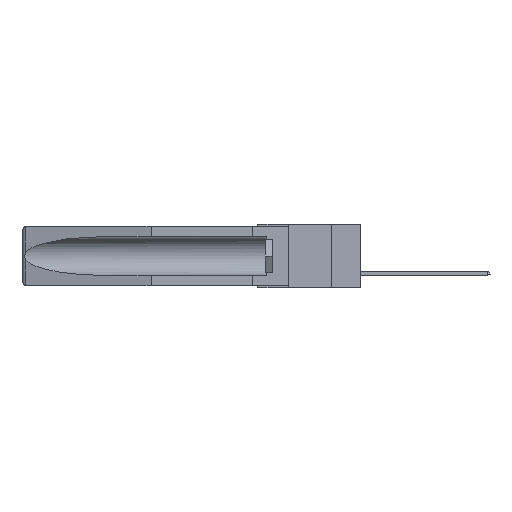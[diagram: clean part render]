
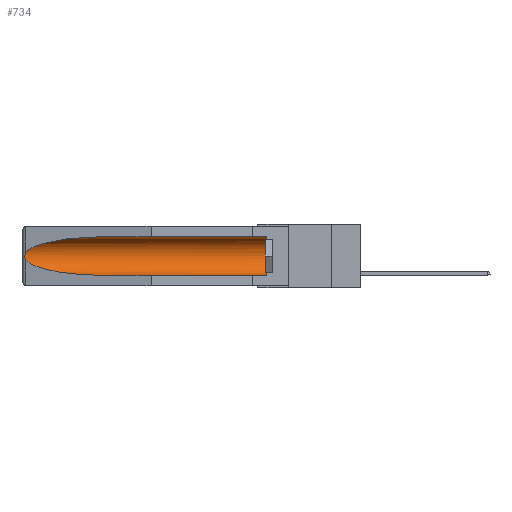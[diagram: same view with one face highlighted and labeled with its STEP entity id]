
A CAD part, left-side view. The second image highlights one B-rep face of the part: STEP entity #734.
In plain terms, the highlighted cylindrical face has radius 2.857 mm (diameter 5.715 mm), a partial arc.
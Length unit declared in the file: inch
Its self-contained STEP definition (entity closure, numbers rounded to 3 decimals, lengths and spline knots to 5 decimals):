
#671 = EDGE_CURVE ( 'NONE', #20543, #9128, #11308, .T. ) ;
#721 = CARTESIAN_POINT ( 'NONE',  ( 0.26537, 1.52718, -0.19328 ) ) ;
#734 = ADVANCED_FACE ( 'NONE', ( #20294 ), #13253, .F. ) ;
#938 = CARTESIAN_POINT ( 'NONE',  ( 0.21114, 1.30732, -0.059 ) ) ;
#1010 =( BOUNDED_CURVE ( )  B_SPLINE_CURVE ( 3, ( #13938, #18757, #17232, #10865 ),
 .UNSPECIFIED., .F., .T. ) 
 B_SPLINE_CURVE_WITH_KNOTS ( ( 4, 4 ),
 ( 0.1948, 1.5708 ),
 .UNSPECIFIED. ) 
 CURVE ( )  GEOMETRIC_REPRESENTATION_ITEM ( )  RATIONAL_B_SPLINE_CURVE ( ( 1., 0.848, 0.848, 1. ) ) 
 REPRESENTATION_ITEM ( '' )  );
#1657 = EDGE_CURVE ( 'NONE', #9608, #5144, #15393, .T. ) ;
#1687 = CARTESIAN_POINT ( 'NONE',  ( 0.26597, 1.52961, -0.15275 ) ) ;
#2240 = CARTESIAN_POINT ( 'NONE',  ( 0.155, -0.30754, -0.1715 ) ) ;
#2378 = VERTEX_POINT ( 'NONE', #11869 ) ;
#2983 = AXIS2_PLACEMENT_3D ( 'NONE', #6679, #3590, #8170 ) ;
#3305 = CARTESIAN_POINT ( 'NONE',  ( 0.26654, 1.53092, -0.15636 ) ) ;
#3590 = DIRECTION ( 'NONE',  ( 0., -1., 0. ) ) ;
#3650 = DIRECTION ( 'NONE',  ( 0., 0., 1. ) ) ;
#3993 = ORIENTED_EDGE ( 'NONE', *, *, #13412, .T. ) ;
#4136 = ORIENTED_EDGE ( 'NONE', *, *, #8612, .F. ) ;
#4415 = CARTESIAN_POINT ( 'NONE',  ( 0.155, -0.30754, -0.284 ) ) ;
#5022 = CIRCLE ( 'NONE', #2983, 0.1125 ) ;
#5144 = VERTEX_POINT ( 'NONE', #10564 ) ;
#6501 = VECTOR ( 'NONE', #14808, 39.37008 ) ;
#6592 = VECTOR ( 'NONE', #14310, 39.37008 ) ;
#6679 = CARTESIAN_POINT ( 'NONE',  ( 0.155, 0.126, -0.1715 ) ) ;
#7323 = ORIENTED_EDGE ( 'NONE', *, *, #671, .T. ) ;
#8170 = DIRECTION ( 'NONE',  ( 0., 0., 1. ) ) ;
#8325 = VERTEX_POINT ( 'NONE', #18918 ) ;
#8612 = EDGE_CURVE ( 'NONE', #8325, #2378, #20167, .T. ) ;
#8706 = CARTESIAN_POINT ( 'NONE',  ( 0.2673, 1.53269, -0.17917 ) ) ;
#9128 = VERTEX_POINT ( 'NONE', #16976 ) ;
#9608 = VERTEX_POINT ( 'NONE', #13157 ) ;
#10125 = CARTESIAN_POINT ( 'NONE',  ( 0.26597, 1.5296, -0.19026 ) ) ;
#10564 = CARTESIAN_POINT ( 'NONE',  ( 0.26537, 1.52718, -0.19328 ) ) ;
#10618 = ORIENTED_EDGE ( 'NONE', *, *, #1657, .T. ) ;
#10779 = EDGE_LOOP ( 'NONE', ( #13760, #10618, #15828, #4136, #3993, #7323 ) ) ;
#10865 = CARTESIAN_POINT ( 'NONE',  ( 0.155, 1.07973, -0.284 ) ) ;
#11308 = LINE ( 'NONE', #11812, #6501 ) ;
#11812 = CARTESIAN_POINT ( 'NONE',  ( 0.155, -0.30754, -0.059 ) ) ;
#11869 = CARTESIAN_POINT ( 'NONE',  ( 0.155, 1.07973, -0.284 ) ) ;
#12294 = CARTESIAN_POINT ( 'NONE',  ( 0.26537, 1.52718, -0.14972 ) ) ;
#13157 = CARTESIAN_POINT ( 'NONE',  ( 0.26537, 1.52718, -0.14972 ) ) ;
#13247 = DIRECTION ( 'NONE',  ( 0., 1., 0. ) ) ;
#13253 = CYLINDRICAL_SURFACE ( 'NONE', #13975, 0.1125 ) ;
#13412 = EDGE_CURVE ( 'NONE', #8325, #20543, #5022, .T. ) ;
#13453 = CARTESIAN_POINT ( 'NONE',  ( 0.2675, 1.53308, -0.16763 ) ) ;
#13527 = CARTESIAN_POINT ( 'NONE',  ( 0.2675, 1.53308, -0.17534 ) ) ;
#13760 = ORIENTED_EDGE ( 'NONE', *, *, #15416, .T. ) ;
#13938 = CARTESIAN_POINT ( 'NONE',  ( 0.26537, 1.52718, -0.19328 ) ) ;
#13967 = CARTESIAN_POINT ( 'NONE',  ( 0.155, 1.07973, -0.059 ) ) ;
#13975 = AXIS2_PLACEMENT_3D ( 'NONE', #2240, #13247, #3650 ) ;
#14310 = DIRECTION ( 'NONE',  ( 0., 1., 0. ) ) ;
#14808 = DIRECTION ( 'NONE',  ( 0., 1., 0. ) ) ;
#15004 =( BOUNDED_CURVE ( )  B_SPLINE_CURVE ( 3, ( #13967, #938, #18649, #12294 ),
 .UNSPECIFIED., .F., .F. ) 
 B_SPLINE_CURVE_WITH_KNOTS ( ( 4, 4 ),
 ( 4.71239, 6.08839 ),
 .UNSPECIFIED. ) 
 CURVE ( )  GEOMETRIC_REPRESENTATION_ITEM ( )  RATIONAL_B_SPLINE_CURVE ( ( 1., 0.848, 0.848, 1. ) ) 
 REPRESENTATION_ITEM ( '' )  );
#15393 = B_SPLINE_CURVE_WITH_KNOTS ( 'NONE', 3,
 ( #19549, #1687, #3305, #16484, #13453, #13527, #8706, #19694, #10125, #721 ),
 .UNSPECIFIED., .F., .F.,
 ( 4, 2, 2, 2, 4 ),
 ( 0., 0.00029, 0.00058, 0.00087, 0.00117 ),
 .UNSPECIFIED. ) ;
#15416 = EDGE_CURVE ( 'NONE', #9128, #9608, #15004, .T. ) ;
#15828 = ORIENTED_EDGE ( 'NONE', *, *, #15908, .T. ) ;
#15908 = EDGE_CURVE ( 'NONE', #5144, #2378, #1010, .T. ) ;
#16484 = CARTESIAN_POINT ( 'NONE',  ( 0.2673, 1.5327, -0.16383 ) ) ;
#16976 = CARTESIAN_POINT ( 'NONE',  ( 0.155, 1.07973, -0.059 ) ) ;
#17232 = CARTESIAN_POINT ( 'NONE',  ( 0.21114, 1.30732, -0.284 ) ) ;
#18649 = CARTESIAN_POINT ( 'NONE',  ( 0.25451, 1.48313, -0.09465 ) ) ;
#18757 = CARTESIAN_POINT ( 'NONE',  ( 0.25451, 1.48313, -0.24835 ) ) ;
#18877 = CARTESIAN_POINT ( 'NONE',  ( 0.155, 0.126, -0.059 ) ) ;
#18918 = CARTESIAN_POINT ( 'NONE',  ( 0.155, 0.126, -0.284 ) ) ;
#19549 = CARTESIAN_POINT ( 'NONE',  ( 0.26537, 1.52718, -0.14972 ) ) ;
#19694 = CARTESIAN_POINT ( 'NONE',  ( 0.26655, 1.53094, -0.18657 ) ) ;
#20167 = LINE ( 'NONE', #4415, #6592 ) ;
#20294 = FACE_OUTER_BOUND ( 'NONE', #10779, .T. ) ;
#20543 = VERTEX_POINT ( 'NONE', #18877 ) ;
